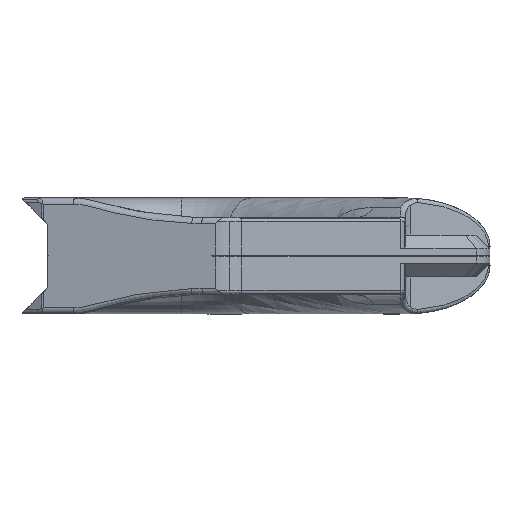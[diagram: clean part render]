
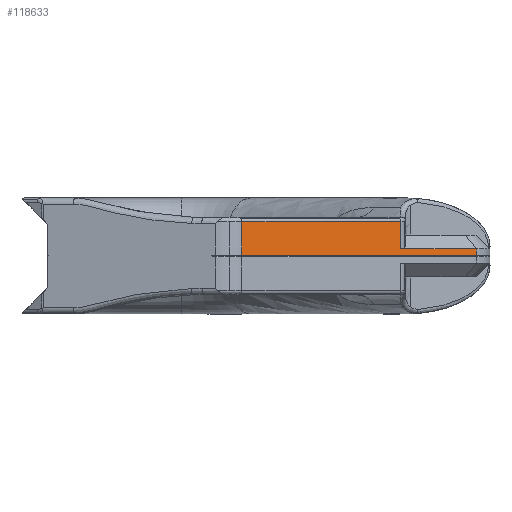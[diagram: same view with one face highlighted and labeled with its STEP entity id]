
A CAD part, left-side view. The second image highlights one B-rep face of the part: STEP entity #118633.
In plain terms, the highlighted planar face has unit normal (-0.772, -0.636, 0).
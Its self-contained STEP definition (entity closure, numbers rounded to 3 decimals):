
#143 = CARTESIAN_POINT ( 'NONE',  ( -61.635, -51.261, 0.5 ) ) ;
#3997 = CARTESIAN_POINT ( 'NONE',  ( -61.635, -51.261, 1.715 ) ) ;
#4725 = LINE ( 'NONE', #251088, #242724 ) ;
#4875 = VERTEX_POINT ( 'NONE', #209369 ) ;
#6050 = DIRECTION ( 'NONE',  ( -0.636, 0.772, 0. ) ) ;
#9221 = CARTESIAN_POINT ( 'NONE',  ( -76.803, -32.838, 8.38 ) ) ;
#16559 = ORIENTED_EDGE ( 'NONE', *, *, #216406, .F. ) ;
#17613 = LINE ( 'NONE', #41927, #50924 ) ;
#17782 = EDGE_CURVE ( 'NONE', #4875, #146215, #227206, .T. ) ;
#20614 = DIRECTION ( 'NONE',  ( -0.636, 0.772, 0. ) ) ;
#24681 = VECTOR ( 'NONE', #220709, 1000. ) ;
#25056 = VERTEX_POINT ( 'NONE', #9221 ) ;
#32097 = VECTOR ( 'NONE', #220093, 1000. ) ;
#34765 = CARTESIAN_POINT ( 'NONE',  ( -61.635, -51.261, 1.715 ) ) ;
#35789 = EDGE_CURVE ( 'NONE', #213071, #257796, #17613, .T. ) ;
#37318 = CARTESIAN_POINT ( 'NONE',  ( -76.803, -32.838, -1.575 ) ) ;
#40752 = DIRECTION ( 'NONE',  ( 0., 0., -1. ) ) ;
#41927 = CARTESIAN_POINT ( 'NONE',  ( -108.579, 5.756, 0.5 ) ) ;
#50924 = VECTOR ( 'NONE', #78547, 1000. ) ;
#51725 = VERTEX_POINT ( 'NONE', #239737 ) ;
#69263 = ORIENTED_EDGE ( 'NONE', *, *, #210567, .F. ) ;
#74040 = ORIENTED_EDGE ( 'NONE', *, *, #241810, .F. ) ;
#78547 = DIRECTION ( 'NONE',  ( 0., 0., -1. ) ) ;
#80034 = LINE ( 'NONE', #143, #92879 ) ;
#82657 = CARTESIAN_POINT ( 'NONE',  ( -104.848, 1.225, 8.377 ) ) ;
#92879 = VECTOR ( 'NONE', #40752, 1000. ) ;
#97346 = CARTESIAN_POINT ( 'NONE',  ( -76.803, -32.838, 1.715 ) ) ;
#104229 = EDGE_CURVE ( 'NONE', #51725, #257796, #4725, .T. ) ;
#109292 = CARTESIAN_POINT ( 'NONE',  ( -108.579, 5.756, 0.2 ) ) ;
#115910 = LINE ( 'NONE', #37318, #32097 ) ;
#118633 = ADVANCED_FACE ( 'NONE', ( #123500 ), #248007, .T. ) ;
#121978 = VECTOR ( 'NONE', #247771, 1000. ) ;
#123500 = FACE_OUTER_BOUND ( 'NONE', #182922, .T. ) ;
#125565 = VERTEX_POINT ( 'NONE', #97346 ) ;
#125924 = ORIENTED_EDGE ( 'NONE', *, *, #251671, .T. ) ;
#127916 = CARTESIAN_POINT ( 'NONE',  ( -108.579, 5.756, 8.376 ) ) ;
#127955 = ORIENTED_EDGE ( 'NONE', *, *, #17782, .F. ) ;
#146215 = VERTEX_POINT ( 'NONE', #34765 ) ;
#147573 = LINE ( 'NONE', #82657, #121978 ) ;
#152547 = ORIENTED_EDGE ( 'NONE', *, *, #104229, .F. ) ;
#153141 = CARTESIAN_POINT ( 'NONE',  ( -86.872, -20.609, 1.715 ) ) ;
#165161 = CARTESIAN_POINT ( 'NONE',  ( -61.641, -51.254, 1.715 ) ) ;
#182922 = EDGE_LOOP ( 'NONE', ( #152547, #69263, #127955, #74040, #125924, #16559, #259813 ) ) ;
#206063 = DIRECTION ( 'NONE',  ( -0.772, -0.636, 0. ) ) ;
#209369 = CARTESIAN_POINT ( 'NONE',  ( -61.641, -51.254, 1.715 ) ) ;
#210567 = EDGE_CURVE ( 'NONE', #146215, #51725, #80034, .T. ) ;
#213071 = VERTEX_POINT ( 'NONE', #127916 ) ;
#216406 = EDGE_CURVE ( 'NONE', #213071, #25056, #147573, .T. ) ;
#220093 = DIRECTION ( 'NONE',  ( 0., 0., 1. ) ) ;
#220709 = DIRECTION ( 'NONE',  ( 0.636, -0.772, 0. ) ) ;
#227206 =( BOUNDED_CURVE ( )  B_SPLINE_CURVE ( 2, ( #165161, #247702, #3997 ),
 .UNSPECIFIED., .F., .F. ) 
 B_SPLINE_CURVE_WITH_KNOTS ( ( 3, 3 ),
 ( 1.668, 1.669 ),
 .UNSPECIFIED. ) 
 CURVE ( )  GEOMETRIC_REPRESENTATION_ITEM ( )  RATIONAL_B_SPLINE_CURVE ( ( 1.091, 1.091, 1.091 ) ) 
 REPRESENTATION_ITEM ( '' )  );
#239737 = CARTESIAN_POINT ( 'NONE',  ( -61.635, -51.261, 0.2 ) ) ;
#241810 = EDGE_CURVE ( 'NONE', #125565, #4875, #261330, .T. ) ;
#242724 = VECTOR ( 'NONE', #6050, 1000. ) ;
#245349 = CARTESIAN_POINT ( 'NONE',  ( -112.36, 10.348, -1.575 ) ) ;
#247001 = AXIS2_PLACEMENT_3D ( 'NONE', #245349, #206063, #20614 ) ;
#247702 = CARTESIAN_POINT ( 'NONE',  ( -61.638, -51.257, 1.715 ) ) ;
#247771 = DIRECTION ( 'NONE',  ( 0.636, -0.772, 0. ) ) ;
#248007 = PLANE ( 'NONE',  #247001 ) ;
#251088 = CARTESIAN_POINT ( 'NONE',  ( -94.602, -11.22, 0.2 ) ) ;
#251671 = EDGE_CURVE ( 'NONE', #125565, #25056, #115910, .T. ) ;
#257796 = VERTEX_POINT ( 'NONE', #109292 ) ;
#259813 = ORIENTED_EDGE ( 'NONE', *, *, #35789, .T. ) ;
#261330 = LINE ( 'NONE', #153141, #24681 ) ;
